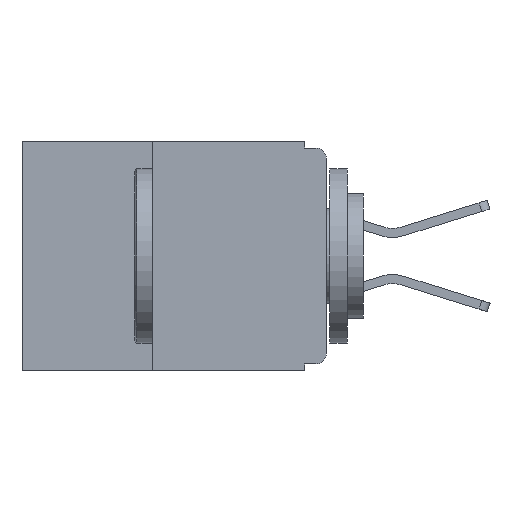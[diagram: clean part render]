
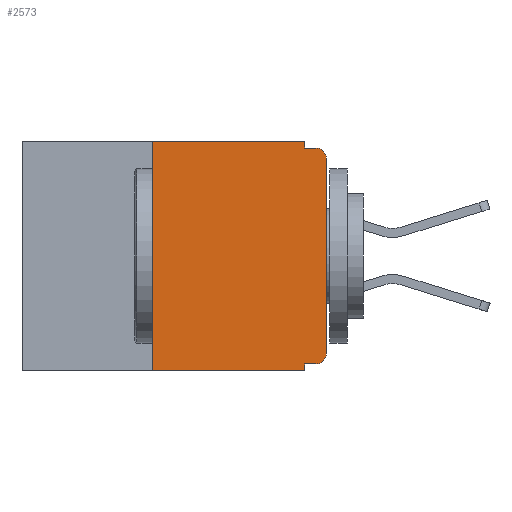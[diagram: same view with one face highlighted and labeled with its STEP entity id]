
A CAD part, left-side view. The second image highlights one B-rep face of the part: STEP entity #2573.
In plain terms, the highlighted planar face has unit normal (-1, 0, 0).
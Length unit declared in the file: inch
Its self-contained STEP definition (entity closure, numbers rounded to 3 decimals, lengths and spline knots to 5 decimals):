
#136 = DIRECTION ( 'NONE',  ( 0., 0., 1. ) ) ;
#379 = AXIS2_PLACEMENT_3D ( 'NONE', #7753, #7522, #7323 ) ;
#500 = VERTEX_POINT ( 'NONE', #10034 ) ;
#672 = VECTOR ( 'NONE', #9458, 39.37008 ) ;
#1222 = EDGE_CURVE ( 'NONE', #1611, #7957, #16519, .T. ) ;
#1611 = VERTEX_POINT ( 'NONE', #4970 ) ;
#1618 = LINE ( 'NONE', #21441, #21081 ) ;
#1881 = EDGE_CURVE ( 'NONE', #17866, #27324, #17375, .T. ) ;
#1943 = EDGE_CURVE ( 'NONE', #22540, #3158, #7760, .T. ) ;
#1996 = CARTESIAN_POINT ( 'NONE',  ( 0., 0.031, -0.33 ) ) ;
#2227 = LINE ( 'NONE', #19108, #24872 ) ;
#2384 = CARTESIAN_POINT ( 'NONE',  ( 0., 0.015, -0.01 ) ) ;
#2573 = ADVANCED_FACE ( 'NONE', ( #16503 ), #7750, .F. ) ;
#3158 = VERTEX_POINT ( 'NONE', #1996 ) ;
#3288 = LINE ( 'NONE', #10029, #30287 ) ;
#3877 = EDGE_CURVE ( 'NONE', #27324, #1611, #2227, .T. ) ;
#4172 = DIRECTION ( 'NONE',  ( 0., -1., 0. ) ) ;
#4721 = CARTESIAN_POINT ( 'NONE',  ( 0., 0.031, 0. ) ) ;
#4912 = ORIENTED_EDGE ( 'NONE', *, *, #1943, .F. ) ;
#4970 = CARTESIAN_POINT ( 'NONE',  ( 0., 0., -0.025 ) ) ;
#6260 = CARTESIAN_POINT ( 'NONE',  ( 0., 0.437, -0.33 ) ) ;
#6406 = CARTESIAN_POINT ( 'NONE',  ( 0., 0.031, -0.32 ) ) ;
#6582 = ORIENTED_EDGE ( 'NONE', *, *, #30362, .F. ) ;
#7297 = VECTOR ( 'NONE', #136, 39.37008 ) ;
#7323 = DIRECTION ( 'NONE',  ( 0., 0., -1. ) ) ;
#7370 = VECTOR ( 'NONE', #29772, 39.37008 ) ;
#7522 = DIRECTION ( 'NONE',  ( 1., 0., 0. ) ) ;
#7750 = PLANE ( 'NONE',  #379 ) ;
#7753 = CARTESIAN_POINT ( 'NONE',  ( 0., 0.437, 0. ) ) ;
#7760 = LINE ( 'NONE', #9742, #672 ) ;
#7957 = VERTEX_POINT ( 'NONE', #2384 ) ;
#9049 = CARTESIAN_POINT ( 'NONE',  ( 0., 0.25, 0. ) ) ;
#9337 = VERTEX_POINT ( 'NONE', #4721 ) ;
#9360 = ORIENTED_EDGE ( 'NONE', *, *, #19015, .F. ) ;
#9458 = DIRECTION ( 'NONE',  ( 0., 0., -1. ) ) ;
#9742 = CARTESIAN_POINT ( 'NONE',  ( 0., 0.031, -0.33 ) ) ;
#10029 = CARTESIAN_POINT ( 'NONE',  ( 0., 0.437, 0. ) ) ;
#10034 = CARTESIAN_POINT ( 'NONE',  ( 0., 0.031, -0.01 ) ) ;
#10865 = EDGE_CURVE ( 'NONE', #17659, #3158, #21418, .T. ) ;
#11066 = VECTOR ( 'NONE', #14741, 39.37008 ) ;
#12091 = CARTESIAN_POINT ( 'NONE',  ( 0., 0., -0.32 ) ) ;
#12151 = CARTESIAN_POINT ( 'NONE',  ( 0., 0., -0.01 ) ) ;
#13449 = ORIENTED_EDGE ( 'NONE', *, *, #10865, .T. ) ;
#14741 = DIRECTION ( 'NONE',  ( 0., 1., 0. ) ) ;
#16333 = DIRECTION ( 'NONE',  ( 0., 0., -1. ) ) ;
#16503 = FACE_OUTER_BOUND ( 'NONE', #16516, .T. ) ;
#16516 = EDGE_LOOP ( 'NONE', ( #24415, #30120, #6582, #25745, #25554, #23279, #13449, #4912, #9360, #30613 ) ) ;
#16519 = CIRCLE ( 'NONE', #19702, 0.015 ) ;
#17357 = EDGE_CURVE ( 'NONE', #9337, #500, #1618, .T. ) ;
#17375 = CIRCLE ( 'NONE', #30413, 0.015 ) ;
#17659 = VERTEX_POINT ( 'NONE', #25097 ) ;
#17866 = VERTEX_POINT ( 'NONE', #25130 ) ;
#18789 = DIRECTION ( 'NONE',  ( 0., 0., 1. ) ) ;
#19015 = EDGE_CURVE ( 'NONE', #17866, #22540, #31645, .T. ) ;
#19108 = CARTESIAN_POINT ( 'NONE',  ( 0., 0., 0. ) ) ;
#19702 = AXIS2_PLACEMENT_3D ( 'NONE', #30053, #33306, #26496 ) ;
#21081 = VECTOR ( 'NONE', #16333, 39.37008 ) ;
#21418 = LINE ( 'NONE', #6260, #7370 ) ;
#21441 = CARTESIAN_POINT ( 'NONE',  ( 0., 0.031, 0. ) ) ;
#22037 = VERTEX_POINT ( 'NONE', #9049 ) ;
#22481 = DIRECTION ( 'NONE',  ( 0., 0., -1. ) ) ;
#22540 = VERTEX_POINT ( 'NONE', #6406 ) ;
#22685 = DIRECTION ( 'NONE',  ( -1., 0., 0. ) ) ;
#22802 = VECTOR ( 'NONE', #4172, 39.37008 ) ;
#23279 = ORIENTED_EDGE ( 'NONE', *, *, #28296, .F. ) ;
#24415 = ORIENTED_EDGE ( 'NONE', *, *, #3877, .T. ) ;
#24430 = CARTESIAN_POINT ( 'NONE',  ( 0., 0.015, -0.305 ) ) ;
#24599 = EDGE_CURVE ( 'NONE', #22037, #9337, #3288, .T. ) ;
#24872 = VECTOR ( 'NONE', #18789, 39.37008 ) ;
#25097 = CARTESIAN_POINT ( 'NONE',  ( 0., 0.25, -0.33 ) ) ;
#25130 = CARTESIAN_POINT ( 'NONE',  ( 0., 0.015, -0.32 ) ) ;
#25554 = ORIENTED_EDGE ( 'NONE', *, *, #24599, .F. ) ;
#25745 = ORIENTED_EDGE ( 'NONE', *, *, #17357, .F. ) ;
#26496 = DIRECTION ( 'NONE',  ( 0., 0., -1. ) ) ;
#26547 = LINE ( 'NONE', #28951, #7297 ) ;
#27324 = VERTEX_POINT ( 'NONE', #27553 ) ;
#27553 = CARTESIAN_POINT ( 'NONE',  ( 0., 0., -0.305 ) ) ;
#28296 = EDGE_CURVE ( 'NONE', #17659, #22037, #26547, .T. ) ;
#28794 = LINE ( 'NONE', #12151, #22802 ) ;
#28951 = CARTESIAN_POINT ( 'NONE',  ( 0., 0.25, -0.33 ) ) ;
#29772 = DIRECTION ( 'NONE',  ( 0., -1., 0. ) ) ;
#30053 = CARTESIAN_POINT ( 'NONE',  ( 0., 0.015, -0.025 ) ) ;
#30120 = ORIENTED_EDGE ( 'NONE', *, *, #1222, .T. ) ;
#30287 = VECTOR ( 'NONE', #30716, 39.37008 ) ;
#30362 = EDGE_CURVE ( 'NONE', #500, #7957, #28794, .T. ) ;
#30413 = AXIS2_PLACEMENT_3D ( 'NONE', #24430, #22685, #22481 ) ;
#30613 = ORIENTED_EDGE ( 'NONE', *, *, #1881, .T. ) ;
#30716 = DIRECTION ( 'NONE',  ( 0., -1., 0. ) ) ;
#31645 = LINE ( 'NONE', #12091, #11066 ) ;
#33306 = DIRECTION ( 'NONE',  ( -1., 0., 0. ) ) ;
